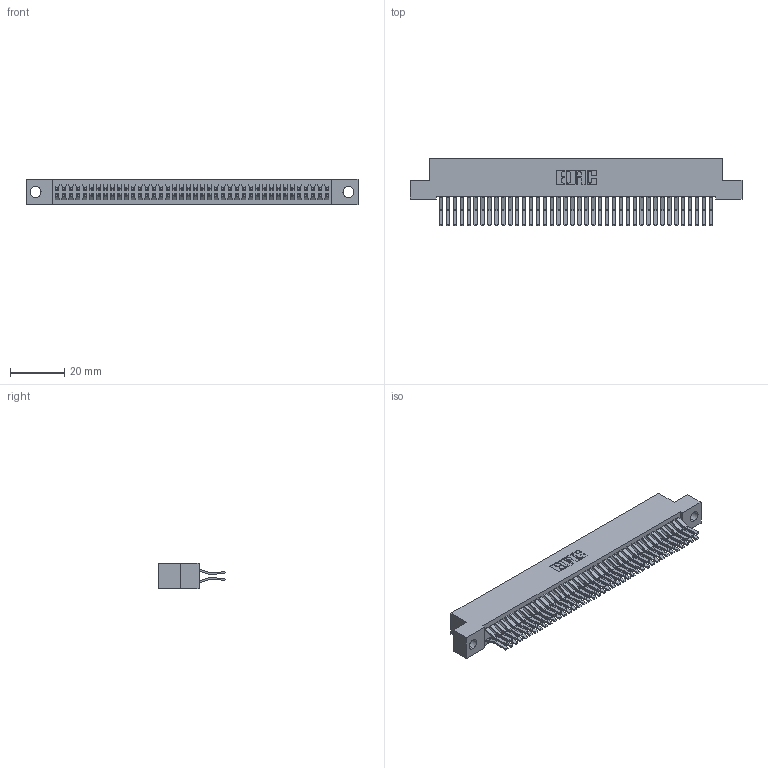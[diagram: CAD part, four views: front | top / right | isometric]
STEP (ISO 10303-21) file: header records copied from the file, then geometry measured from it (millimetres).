
FILE_DESCRIPTION (( 'STEP AP203' ), '1' );
FILE_NAME ('392-080-560-204.STEP', '2018-08-18T03:21:37', ( '' ), ( '' ), 'SwSTEP 2.0', 'SolidWorks 2016', '' );
FILE_SCHEMA (( 'CONFIG_CONTROL_DESIGN' ));
Length unit declared in the file: inch
Products named in the file (3): 342 Part_.156 TH; 345-292-001_560 Tail; 392-080-560-204
Assembly tree (81 placements, depth 2):
  392-080-560-204
    342 Part_.156 TH
    345-292-001_560 Tail  x80
Bounding box: 121.92 x 24.78 x 9.4 mm (x, y, z)
Volume: 11383.2 mm3; surface area: 19563.4 mm2
Topology: 81 solids, 81 shells, 4430 faces, 13179 edges, 8678 vertices
Faces by surface type: plane 2946, cylinder 1484
Entity records: 25951 total; most frequent: CARTESIAN_POINT 4302, ORIENTED_EDGE 4238, DIRECTION 3683, EDGE_CURVE 2119, LINE 1987, VECTOR 1987, VERTEX_POINT 1410, AXIS2_PLACEMENT_3D 848
